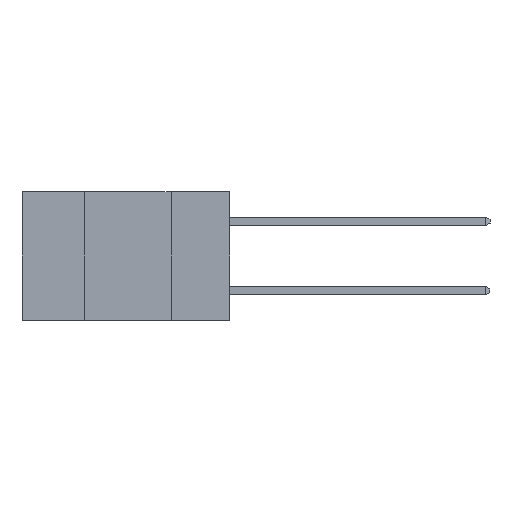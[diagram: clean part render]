
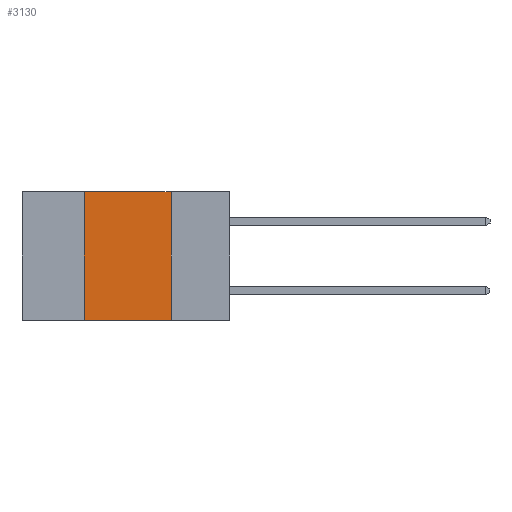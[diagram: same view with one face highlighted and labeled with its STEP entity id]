
A CAD part, left-side view. The second image highlights one B-rep face of the part: STEP entity #3130.
In plain terms, the highlighted planar face has unit normal (-1, 0, 0).
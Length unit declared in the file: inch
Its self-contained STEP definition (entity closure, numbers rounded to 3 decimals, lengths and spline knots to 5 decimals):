
#11 = AXIS2_PLACEMENT_3D ( 'NONE', #15148, #11955, #15021 ) ;
#270 = VERTEX_POINT ( 'NONE', #4656 ) ;
#410 = ORIENTED_EDGE ( 'NONE', *, *, #10879, .F. ) ;
#1370 = CARTESIAN_POINT ( 'NONE',  ( 0., 0.42, 0. ) ) ;
#2702 = VERTEX_POINT ( 'NONE', #11762 ) ;
#3130 = ADVANCED_FACE ( 'NONE', ( #14853 ), #9295, .F. ) ;
#3142 = DIRECTION ( 'NONE',  ( 0., 0., -1. ) ) ;
#3336 = VECTOR ( 'NONE', #13394, 39.37008 ) ;
#4027 = CARTESIAN_POINT ( 'NONE',  ( 0., 0.17, 0. ) ) ;
#4320 = ORIENTED_EDGE ( 'NONE', *, *, #4960, .T. ) ;
#4372 = EDGE_CURVE ( 'NONE', #9542, #12544, #13581, .T. ) ;
#4656 = CARTESIAN_POINT ( 'NONE',  ( 0., 0.42, -0.37 ) ) ;
#4960 = EDGE_CURVE ( 'NONE', #270, #2702, #8765, .T. ) ;
#5783 = LINE ( 'NONE', #13865, #15110 ) ;
#5995 = ORIENTED_EDGE ( 'NONE', *, *, #6594, .F. ) ;
#6594 = EDGE_CURVE ( 'NONE', #270, #9542, #5783, .T. ) ;
#6840 = CARTESIAN_POINT ( 'NONE',  ( 0., 0.6, 0. ) ) ;
#8765 = LINE ( 'NONE', #13443, #12135 ) ;
#9295 = PLANE ( 'NONE',  #11 ) ;
#9313 = CARTESIAN_POINT ( 'NONE',  ( 0., 0.17, 0. ) ) ;
#9542 = VERTEX_POINT ( 'NONE', #1370 ) ;
#10279 = ORIENTED_EDGE ( 'NONE', *, *, #4372, .F. ) ;
#10879 = EDGE_CURVE ( 'NONE', #12544, #2702, #15195, .T. ) ;
#11762 = CARTESIAN_POINT ( 'NONE',  ( 0., 0.17, -0.37 ) ) ;
#11955 = DIRECTION ( 'NONE',  ( 1., 0., 0. ) ) ;
#12135 = VECTOR ( 'NONE', #13421, 39.37008 ) ;
#12159 = VECTOR ( 'NONE', #3142, 39.37008 ) ;
#12544 = VERTEX_POINT ( 'NONE', #4027 ) ;
#13394 = DIRECTION ( 'NONE',  ( 0., -1., 0. ) ) ;
#13421 = DIRECTION ( 'NONE',  ( 0., -1., 0. ) ) ;
#13443 = CARTESIAN_POINT ( 'NONE',  ( 0., 0.6, -0.37 ) ) ;
#13581 = LINE ( 'NONE', #6840, #3336 ) ;
#13757 = DIRECTION ( 'NONE',  ( 0., 0., 1. ) ) ;
#13865 = CARTESIAN_POINT ( 'NONE',  ( 0., 0.42, 0. ) ) ;
#14853 = FACE_OUTER_BOUND ( 'NONE', #15479, .T. ) ;
#15021 = DIRECTION ( 'NONE',  ( 0., 0., -1. ) ) ;
#15110 = VECTOR ( 'NONE', #13757, 39.37008 ) ;
#15148 = CARTESIAN_POINT ( 'NONE',  ( 0., 0.6, 0. ) ) ;
#15195 = LINE ( 'NONE', #9313, #12159 ) ;
#15479 = EDGE_LOOP ( 'NONE', ( #410, #10279, #5995, #4320 ) ) ;
